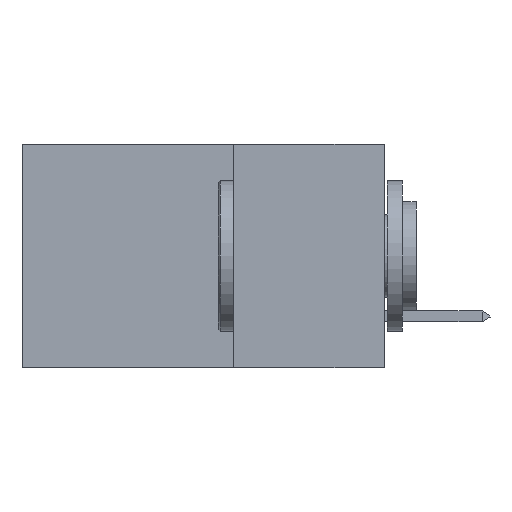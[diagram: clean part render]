
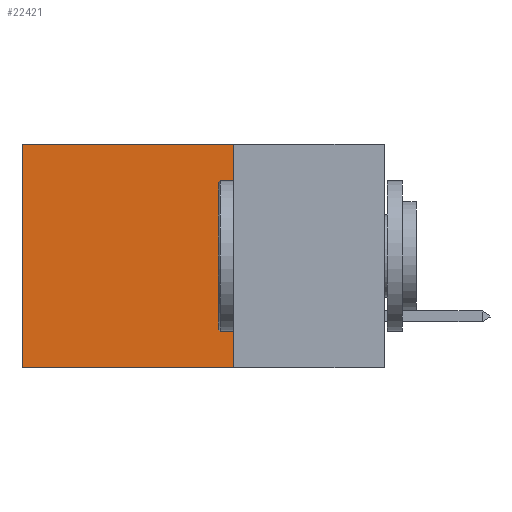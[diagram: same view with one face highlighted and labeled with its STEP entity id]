
A CAD part, left-side view. The second image highlights one B-rep face of the part: STEP entity #22421.
In plain terms, the highlighted planar face has unit normal (-1, 0, 0).
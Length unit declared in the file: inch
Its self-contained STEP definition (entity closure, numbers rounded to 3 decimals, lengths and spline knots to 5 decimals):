
#103 = LINE ( 'NONE', #599, #15076 ) ;
#291 = EDGE_CURVE ( 'NONE', #19788, #19102, #15695, .T. ) ;
#599 = CARTESIAN_POINT ( 'NONE',  ( 0.2875, 0.25, 0. ) ) ;
#1761 = CARTESIAN_POINT ( 'NONE',  ( 0.2875, 0.25, 0. ) ) ;
#1833 = DIRECTION ( 'NONE',  ( 0., 0., -1. ) ) ;
#1972 = EDGE_CURVE ( 'NONE', #19102, #10778, #17236, .T. ) ;
#2356 = FACE_OUTER_BOUND ( 'NONE', #10993, .T. ) ;
#2723 = ORIENTED_EDGE ( 'NONE', *, *, #291, .F. ) ;
#5762 = EDGE_CURVE ( 'NONE', #19788, #12775, #103, .T. ) ;
#5860 = VECTOR ( 'NONE', #16506, 39.37008 ) ;
#5961 = DIRECTION ( 'NONE',  ( 0., 1., 0. ) ) ;
#6207 = DIRECTION ( 'NONE',  ( 0., 0., -1. ) ) ;
#6248 = CARTESIAN_POINT ( 'NONE',  ( 0.2875, 0.6, 0. ) ) ;
#7819 = CARTESIAN_POINT ( 'NONE',  ( 0.2875, 0.25, -0.37 ) ) ;
#8823 = CARTESIAN_POINT ( 'NONE',  ( 0.2875, 0.25, 0. ) ) ;
#8928 = LINE ( 'NONE', #18399, #12155 ) ;
#9560 = EDGE_CURVE ( 'NONE', #12775, #10778, #8928, .T. ) ;
#10716 = CARTESIAN_POINT ( 'NONE',  ( 0.2875, 0.25, -0.37 ) ) ;
#10778 = VERTEX_POINT ( 'NONE', #11032 ) ;
#10993 = EDGE_LOOP ( 'NONE', ( #18882, #13738, #2723, #15854 ) ) ;
#11032 = CARTESIAN_POINT ( 'NONE',  ( 0.2875, 0.6, -0.37 ) ) ;
#12155 = VECTOR ( 'NONE', #6207, 39.37008 ) ;
#12775 = VERTEX_POINT ( 'NONE', #6248 ) ;
#13738 = ORIENTED_EDGE ( 'NONE', *, *, #1972, .F. ) ;
#14025 = VECTOR ( 'NONE', #1833, 39.37008 ) ;
#15076 = VECTOR ( 'NONE', #5961, 39.37008 ) ;
#15695 = LINE ( 'NONE', #17762, #14025 ) ;
#15854 = ORIENTED_EDGE ( 'NONE', *, *, #5762, .T. ) ;
#16506 = DIRECTION ( 'NONE',  ( 0., 1., 0. ) ) ;
#17236 = LINE ( 'NONE', #7819, #5860 ) ;
#17535 = DIRECTION ( 'NONE',  ( 0., 0., -1. ) ) ;
#17762 = CARTESIAN_POINT ( 'NONE',  ( 0.2875, 0.25, 0. ) ) ;
#18399 = CARTESIAN_POINT ( 'NONE',  ( 0.2875, 0.6, 0. ) ) ;
#18882 = ORIENTED_EDGE ( 'NONE', *, *, #9560, .T. ) ;
#19102 = VERTEX_POINT ( 'NONE', #10716 ) ;
#19112 = DIRECTION ( 'NONE',  ( 1., 0., 0. ) ) ;
#19334 = PLANE ( 'NONE',  #20990 ) ;
#19788 = VERTEX_POINT ( 'NONE', #1761 ) ;
#20990 = AXIS2_PLACEMENT_3D ( 'NONE', #8823, #19112, #17535 ) ;
#22421 = ADVANCED_FACE ( 'NONE', ( #2356 ), #19334, .F. ) ;
